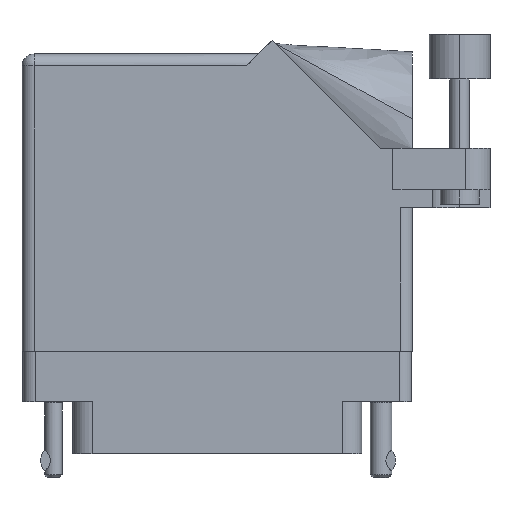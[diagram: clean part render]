
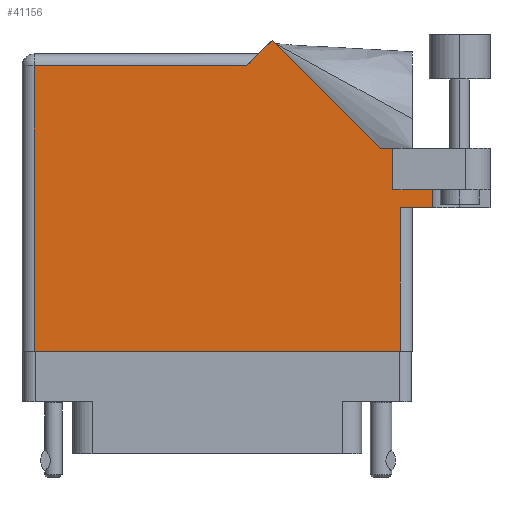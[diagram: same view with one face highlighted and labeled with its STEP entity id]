
A CAD part, front view. The second image highlights one B-rep face of the part: STEP entity #41156.
In plain terms, the highlighted face is planar.
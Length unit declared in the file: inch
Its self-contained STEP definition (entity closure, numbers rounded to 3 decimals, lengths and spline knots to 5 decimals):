
#1235 = DIRECTION ( 'NONE',  ( -1., 0., 0. ) ) ;
#1447 = ORIENTED_EDGE ( 'NONE', *, *, #33321, .F. ) ;
#1464 = EDGE_CURVE ( 'NONE', #42663, #10090, #9091, .T. ) ;
#1705 = ORIENTED_EDGE ( 'NONE', *, *, #29600, .T. ) ;
#4005 = CARTESIAN_POINT ( 'NONE',  ( 2.1115, 1.16177, 0. ) ) ;
#4535 = EDGE_CURVE ( 'NONE', #38401, #34947, #6534, .T. ) ;
#4558 = ORIENTED_EDGE ( 'NONE', *, *, #1464, .T. ) ;
#4927 = DIRECTION ( 'NONE',  ( 0., -1., 0. ) ) ;
#5248 = ORIENTED_EDGE ( 'NONE', *, *, #4535, .F. ) ;
#5803 = CARTESIAN_POINT ( 'NONE',  ( 1.155, 1.468, 0. ) ) ;
#6155 = DIRECTION ( 'NONE',  ( -1., 0., 0. ) ) ;
#6534 = LINE ( 'NONE', #4005, #30032 ) ;
#6590 = CARTESIAN_POINT ( 'NONE',  ( 1.91, 0.831, 0. ) ) ;
#7034 = FACE_OUTER_BOUND ( 'NONE', #33190, .T. ) ;
#7964 = CARTESIAN_POINT ( 'NONE',  ( 1.84442, 1.044, 0. ) ) ;
#9091 = LINE ( 'NONE', #30080, #31981 ) ;
#9291 = DIRECTION ( 'NONE',  ( -0.707, 0.707, 0. ) ) ;
#10090 = VERTEX_POINT ( 'NONE', #5803 ) ;
#10118 = CARTESIAN_POINT ( 'NONE',  ( 2.1115, 0.831, 0. ) ) ;
#10837 = VECTOR ( 'NONE', #41585, 39.37008 ) ;
#11040 = VERTEX_POINT ( 'NONE', #47717 ) ;
#11126 = CARTESIAN_POINT ( 'NONE',  ( 0.062, 1.468, 0. ) ) ;
#11975 = VECTOR ( 'NONE', #26561, 39.37008 ) ;
#12266 = VECTOR ( 'NONE', #13831, 39.37008 ) ;
#12481 = CARTESIAN_POINT ( 'NONE',  ( 0., 1.53, 0. ) ) ;
#13655 = VERTEX_POINT ( 'NONE', #36889 ) ;
#13831 = DIRECTION ( 'NONE',  ( 0., 1., 0. ) ) ;
#15340 = CARTESIAN_POINT ( 'NONE',  ( 1.91, 0.831, 0. ) ) ;
#15809 = ORIENTED_EDGE ( 'NONE', *, *, #35806, .T. ) ;
#16225 = DIRECTION ( 'NONE',  ( 0., 0., -1. ) ) ;
#17931 = VECTOR ( 'NONE', #39762, 39.37008 ) ;
#18674 = EDGE_CURVE ( 'NONE', #25110, #42663, #29351, .T. ) ;
#19266 = DIRECTION ( 'NONE',  ( 1., 0., 0. ) ) ;
#19709 = CARTESIAN_POINT ( 'NONE',  ( 0., 1.468, 0. ) ) ;
#19950 = CARTESIAN_POINT ( 'NONE',  ( 0.062, 0., 0. ) ) ;
#20785 = ORIENTED_EDGE ( 'NONE', *, *, #23226, .T. ) ;
#21559 = CARTESIAN_POINT ( 'NONE',  ( 2.01, 0.737, 0. ) ) ;
#23029 = DIRECTION ( 'NONE',  ( -1., 0., 0. ) ) ;
#23226 = EDGE_CURVE ( 'NONE', #11040, #13655, #37248, .T. ) ;
#23376 = ORIENTED_EDGE ( 'NONE', *, *, #18674, .T. ) ;
#23405 = VECTOR ( 'NONE', #4927, 39.37008 ) ;
#24351 = LINE ( 'NONE', #41010, #11975 ) ;
#24741 = VECTOR ( 'NONE', #19266, 39.37008 ) ;
#25110 = VERTEX_POINT ( 'NONE', #7964 ) ;
#26486 = CARTESIAN_POINT ( 'NONE',  ( 0., 0., 0. ) ) ;
#26561 = DIRECTION ( 'NONE',  ( 0., 1., 0. ) ) ;
#27750 = EDGE_CURVE ( 'NONE', #43860, #11040, #44002, .T. ) ;
#29250 = ORIENTED_EDGE ( 'NONE', *, *, #27750, .T. ) ;
#29351 = LINE ( 'NONE', #46648, #35747 ) ;
#29600 = EDGE_CURVE ( 'NONE', #48530, #34947, #43814, .T. ) ;
#30032 = VECTOR ( 'NONE', #37753, 39.37008 ) ;
#30080 = CARTESIAN_POINT ( 'NONE',  ( 1.217, 1.53, 0. ) ) ;
#30537 = VERTEX_POINT ( 'NONE', #38201 ) ;
#30756 = AXIS2_PLACEMENT_3D ( 'NONE', #12481, #16225, #1235 ) ;
#31981 = VECTOR ( 'NONE', #41190, 39.37008 ) ;
#32742 = EDGE_CURVE ( 'NONE', #35670, #30537, #24351, .T. ) ;
#33190 = EDGE_LOOP ( 'NONE', ( #20785, #15809, #1705, #5248, #1447, #41622, #38667, #23376, #4558, #43253, #29250 ) ) ;
#33321 = EDGE_CURVE ( 'NONE', #35670, #38401, #34718, .T. ) ;
#34718 = LINE ( 'NONE', #15340, #24741 ) ;
#34947 = VERTEX_POINT ( 'NONE', #47579 ) ;
#35670 = VERTEX_POINT ( 'NONE', #6590 ) ;
#35747 = VECTOR ( 'NONE', #9291, 39.37008 ) ;
#35806 = EDGE_CURVE ( 'NONE', #13655, #48530, #42784, .T. ) ;
#35855 = CARTESIAN_POINT ( 'NONE',  ( 1.948, 0.737, 0. ) ) ;
#36889 = CARTESIAN_POINT ( 'NONE',  ( 1.948, 0., 0. ) ) ;
#37248 = LINE ( 'NONE', #26486, #10837 ) ;
#37753 = DIRECTION ( 'NONE',  ( 0., -1., 0. ) ) ;
#38201 = CARTESIAN_POINT ( 'NONE',  ( 1.91, 1.044, 0. ) ) ;
#38397 = PLANE ( 'NONE',  #30756 ) ;
#38401 = VERTEX_POINT ( 'NONE', #10118 ) ;
#38667 = ORIENTED_EDGE ( 'NONE', *, *, #47344, .T. ) ;
#39472 = LINE ( 'NONE', #19709, #45932 ) ;
#39561 = CARTESIAN_POINT ( 'NONE',  ( 2.41, 1.044, 0. ) ) ;
#39762 = DIRECTION ( 'NONE',  ( 1., 0., 0. ) ) ;
#39972 = EDGE_CURVE ( 'NONE', #10090, #43860, #39472, .T. ) ;
#39993 = VECTOR ( 'NONE', #6155, 39.37008 ) ;
#41010 = CARTESIAN_POINT ( 'NONE',  ( 1.91, 0.831, 0. ) ) ;
#41113 = CARTESIAN_POINT ( 'NONE',  ( 1.948, 0.737, 0. ) ) ;
#41156 = ADVANCED_FACE ( 'NONE', ( #7034 ), #38397, .F. ) ;
#41190 = DIRECTION ( 'NONE',  ( -0.707, -0.707, 0. ) ) ;
#41585 = DIRECTION ( 'NONE',  ( 1., 0., 0. ) ) ;
#41622 = ORIENTED_EDGE ( 'NONE', *, *, #32742, .T. ) ;
#42663 = VERTEX_POINT ( 'NONE', #47152 ) ;
#42784 = LINE ( 'NONE', #35855, #12266 ) ;
#43253 = ORIENTED_EDGE ( 'NONE', *, *, #39972, .T. ) ;
#43814 = LINE ( 'NONE', #21559, #17931 ) ;
#43860 = VERTEX_POINT ( 'NONE', #11126 ) ;
#44002 = LINE ( 'NONE', #19950, #23405 ) ;
#45932 = VECTOR ( 'NONE', #23029, 39.37008 ) ;
#46437 = LINE ( 'NONE', #39561, #39993 ) ;
#46648 = CARTESIAN_POINT ( 'NONE',  ( 1.84442, 1.044, 0. ) ) ;
#47152 = CARTESIAN_POINT ( 'NONE',  ( 1.28771, 1.60071, 0. ) ) ;
#47344 = EDGE_CURVE ( 'NONE', #30537, #25110, #46437, .T. ) ;
#47579 = CARTESIAN_POINT ( 'NONE',  ( 2.1115, 0.737, 0. ) ) ;
#47717 = CARTESIAN_POINT ( 'NONE',  ( 0.062, 0., 0. ) ) ;
#48530 = VERTEX_POINT ( 'NONE', #41113 ) ;
